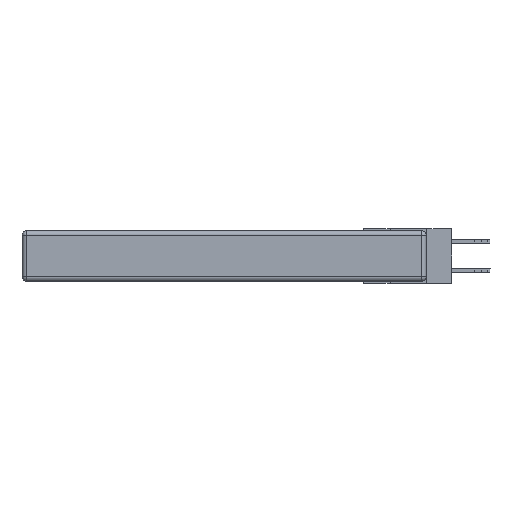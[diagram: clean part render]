
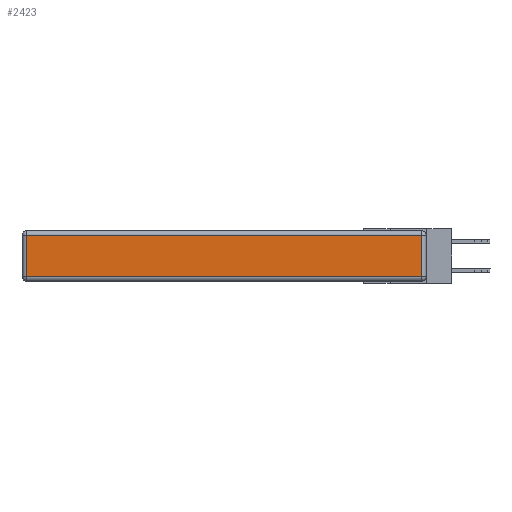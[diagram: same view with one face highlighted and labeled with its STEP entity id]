
A CAD part, left-side view. The second image highlights one B-rep face of the part: STEP entity #2423.
In plain terms, the highlighted planar face has unit normal (-1, 0, 0).
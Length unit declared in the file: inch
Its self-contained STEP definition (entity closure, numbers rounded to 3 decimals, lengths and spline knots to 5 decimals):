
#190 = VECTOR ( 'NONE', #12342, 39.37008 ) ;
#425 = VERTEX_POINT ( 'NONE', #9449 ) ;
#683 = ORIENTED_EDGE ( 'NONE', *, *, #3384, .T. ) ;
#788 = EDGE_CURVE ( 'NONE', #425, #9488, #11987, .T. ) ;
#978 = LINE ( 'NONE', #10508, #2747 ) ;
#1618 = CARTESIAN_POINT ( 'NONE',  ( 0., 0., -0.313 ) ) ;
#1960 = ORIENTED_EDGE ( 'NONE', *, *, #2849, .T. ) ;
#2082 = VERTEX_POINT ( 'NONE', #8405 ) ;
#2423 = ADVANCED_FACE ( 'NONE', ( #9291 ), #9495, .T. ) ;
#2722 = LINE ( 'NONE', #1618, #7353 ) ;
#2747 = VECTOR ( 'NONE', #11605, 39.37008 ) ;
#2849 = EDGE_CURVE ( 'NONE', #9327, #2082, #2722, .T. ) ;
#3090 = DIRECTION ( 'NONE',  ( 0., 1., 0. ) ) ;
#3237 = CARTESIAN_POINT ( 'NONE',  ( 0., 2.72, -0.313 ) ) ;
#3384 = EDGE_CURVE ( 'NONE', #2082, #425, #978, .T. ) ;
#3743 = LINE ( 'NONE', #5562, #190 ) ;
#3901 = DIRECTION ( 'NONE',  ( 0., 0., 1. ) ) ;
#4554 = ORIENTED_EDGE ( 'NONE', *, *, #6691, .T. ) ;
#4709 = VECTOR ( 'NONE', #3090, 39.37008 ) ;
#5562 = CARTESIAN_POINT ( 'NONE',  ( 0., 2.72, -0.343 ) ) ;
#6189 = DIRECTION ( 'NONE',  ( 0., -1., 0. ) ) ;
#6691 = EDGE_CURVE ( 'NONE', #9488, #9327, #3743, .T. ) ;
#7192 = AXIS2_PLACEMENT_3D ( 'NONE', #10743, #7334, #3901 ) ;
#7334 = DIRECTION ( 'NONE',  ( -1., 0., 0. ) ) ;
#7353 = VECTOR ( 'NONE', #6189, 39.37008 ) ;
#8088 = CARTESIAN_POINT ( 'NONE',  ( 0., 2.72, -0.03 ) ) ;
#8405 = CARTESIAN_POINT ( 'NONE',  ( 0., 0.03, -0.313 ) ) ;
#8735 = CARTESIAN_POINT ( 'NONE',  ( 0., 2.75, -0.03 ) ) ;
#9137 = ORIENTED_EDGE ( 'NONE', *, *, #788, .T. ) ;
#9291 = FACE_OUTER_BOUND ( 'NONE', #11645, .T. ) ;
#9327 = VERTEX_POINT ( 'NONE', #3237 ) ;
#9449 = CARTESIAN_POINT ( 'NONE',  ( 0., 0.03, -0.03 ) ) ;
#9488 = VERTEX_POINT ( 'NONE', #8088 ) ;
#9495 = PLANE ( 'NONE',  #7192 ) ;
#10508 = CARTESIAN_POINT ( 'NONE',  ( 0., 0.03, -0.343 ) ) ;
#10743 = CARTESIAN_POINT ( 'NONE',  ( 0., 0., -0.343 ) ) ;
#11605 = DIRECTION ( 'NONE',  ( 0., 0., 1. ) ) ;
#11645 = EDGE_LOOP ( 'NONE', ( #1960, #683, #9137, #4554 ) ) ;
#11987 = LINE ( 'NONE', #8735, #4709 ) ;
#12342 = DIRECTION ( 'NONE',  ( 0., 0., -1. ) ) ;
